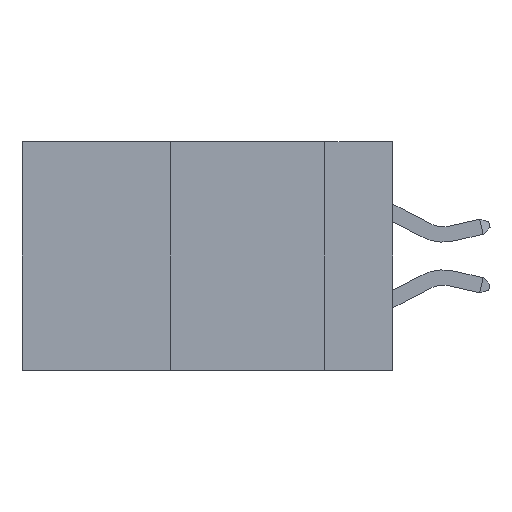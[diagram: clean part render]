
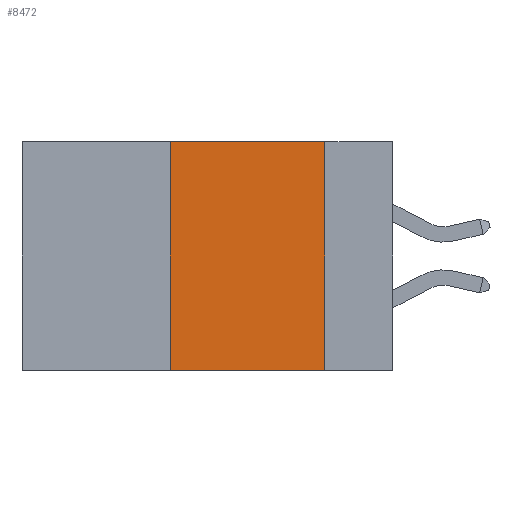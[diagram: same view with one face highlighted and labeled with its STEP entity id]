
A CAD part, left-side view. The second image highlights one B-rep face of the part: STEP entity #8472.
In plain terms, the highlighted planar face has unit normal (-1, 0, 0).
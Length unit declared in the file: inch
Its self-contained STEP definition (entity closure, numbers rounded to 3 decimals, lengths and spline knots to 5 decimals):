
#972 = ORIENTED_EDGE ( 'NONE', *, *, #8756, .F. ) ;
#2260 = CARTESIAN_POINT ( 'NONE',  ( 0., 0.6, 0. ) ) ;
#2767 = ORIENTED_EDGE ( 'NONE', *, *, #18092, .F. ) ;
#2983 = AXIS2_PLACEMENT_3D ( 'NONE', #7447, #23937, #11470 ) ;
#3862 = VECTOR ( 'NONE', #22558, 39.37008 ) ;
#4045 = CARTESIAN_POINT ( 'NONE',  ( 0., 0.36, 0. ) ) ;
#5470 = PLANE ( 'NONE',  #2983 ) ;
#5607 = EDGE_CURVE ( 'NONE', #15417, #20713, #8098, .T. ) ;
#6737 = VERTEX_POINT ( 'NONE', #4045 ) ;
#7447 = CARTESIAN_POINT ( 'NONE',  ( 0., 0.6, 0. ) ) ;
#7565 = LINE ( 'NONE', #18616, #17225 ) ;
#8098 = LINE ( 'NONE', #10143, #11950 ) ;
#8431 = CARTESIAN_POINT ( 'NONE',  ( 0., 0.11, 0. ) ) ;
#8472 = ADVANCED_FACE ( 'NONE', ( #13707 ), #5470, .F. ) ;
#8756 = EDGE_CURVE ( 'NONE', #15261, #20713, #7565, .T. ) ;
#10143 = CARTESIAN_POINT ( 'NONE',  ( 0., 0.6, -0.37 ) ) ;
#11470 = DIRECTION ( 'NONE',  ( 0., 0., -1. ) ) ;
#11950 = VECTOR ( 'NONE', #26074, 39.37008 ) ;
#12343 = ORIENTED_EDGE ( 'NONE', *, *, #5607, .T. ) ;
#12423 = CARTESIAN_POINT ( 'NONE',  ( 0., 0.11, -0.37 ) ) ;
#12529 = VECTOR ( 'NONE', #20529, 39.37008 ) ;
#12915 = EDGE_CURVE ( 'NONE', #6737, #15261, #19633, .T. ) ;
#13155 = ORIENTED_EDGE ( 'NONE', *, *, #12915, .F. ) ;
#13366 = CARTESIAN_POINT ( 'NONE',  ( 0., 0.36, 0. ) ) ;
#13707 = FACE_OUTER_BOUND ( 'NONE', #17105, .T. ) ;
#14443 = LINE ( 'NONE', #13366, #12529 ) ;
#15261 = VERTEX_POINT ( 'NONE', #8431 ) ;
#15417 = VERTEX_POINT ( 'NONE', #18022 ) ;
#16343 = DIRECTION ( 'NONE',  ( 0., 0., -1. ) ) ;
#17105 = EDGE_LOOP ( 'NONE', ( #972, #13155, #2767, #12343 ) ) ;
#17225 = VECTOR ( 'NONE', #16343, 39.37008 ) ;
#18022 = CARTESIAN_POINT ( 'NONE',  ( 0., 0.36, -0.37 ) ) ;
#18092 = EDGE_CURVE ( 'NONE', #15417, #6737, #14443, .T. ) ;
#18616 = CARTESIAN_POINT ( 'NONE',  ( 0., 0.11, 0. ) ) ;
#19633 = LINE ( 'NONE', #2260, #3862 ) ;
#20529 = DIRECTION ( 'NONE',  ( 0., 0., 1. ) ) ;
#20713 = VERTEX_POINT ( 'NONE', #12423 ) ;
#22558 = DIRECTION ( 'NONE',  ( 0., -1., 0. ) ) ;
#23937 = DIRECTION ( 'NONE',  ( 1., 0., 0. ) ) ;
#26074 = DIRECTION ( 'NONE',  ( 0., -1., 0. ) ) ;
